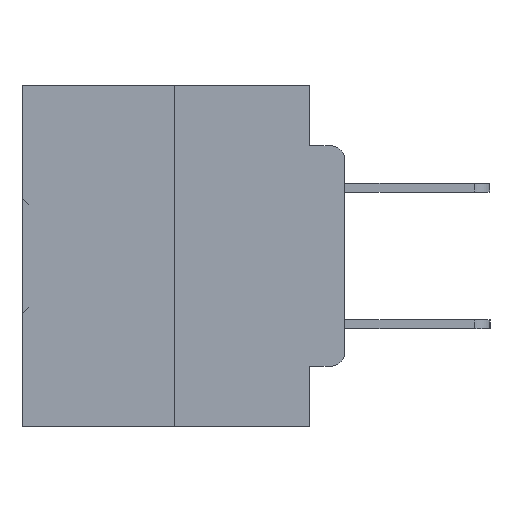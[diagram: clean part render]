
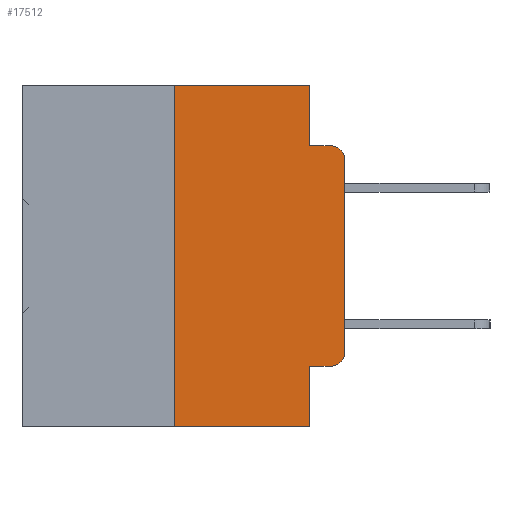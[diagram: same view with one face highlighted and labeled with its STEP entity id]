
A CAD part, left-side view. The second image highlights one B-rep face of the part: STEP entity #17512.
In plain terms, the highlighted planar face has unit normal (-1, 0, 0).
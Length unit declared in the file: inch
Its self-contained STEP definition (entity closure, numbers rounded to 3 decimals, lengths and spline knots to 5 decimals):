
#253 = VERTEX_POINT ( 'NONE', #17229 ) ;
#1044 = LINE ( 'NONE', #12478, #2604 ) ;
#1813 = DIRECTION ( 'NONE',  ( 0., 0., -1. ) ) ;
#1970 = VERTEX_POINT ( 'NONE', #19593 ) ;
#2037 = CARTESIAN_POINT ( 'NONE',  ( 0., 0.473, -0.5 ) ) ;
#2222 = DIRECTION ( 'NONE',  ( 0., 0., -1. ) ) ;
#2604 = VECTOR ( 'NONE', #35275, 39.37008 ) ;
#2745 = ORIENTED_EDGE ( 'NONE', *, *, #32824, .F. ) ;
#3114 = VECTOR ( 'NONE', #10471, 39.37008 ) ;
#3212 = CIRCLE ( 'NONE', #5008, 0.02 ) ;
#3658 = VERTEX_POINT ( 'NONE', #12360 ) ;
#3926 = CARTESIAN_POINT ( 'NONE',  ( 0., 0.473, 0. ) ) ;
#4075 = VERTEX_POINT ( 'NONE', #29695 ) ;
#4568 = VERTEX_POINT ( 'NONE', #26254 ) ;
#5008 = AXIS2_PLACEMENT_3D ( 'NONE', #9874, #18976, #12669 ) ;
#5252 = VECTOR ( 'NONE', #19465, 39.37008 ) ;
#5935 = CARTESIAN_POINT ( 'NONE',  ( 0., 0.051, 0. ) ) ;
#6738 = DIRECTION ( 'NONE',  ( 0., -1., 0. ) ) ;
#6985 = VERTEX_POINT ( 'NONE', #8319 ) ;
#7300 = ORIENTED_EDGE ( 'NONE', *, *, #29198, .F. ) ;
#7474 = DIRECTION ( 'NONE',  ( -1., 0., 0. ) ) ;
#7895 = DIRECTION ( 'NONE',  ( 0., -1., 0. ) ) ;
#8212 = LINE ( 'NONE', #5935, #25805 ) ;
#8319 = CARTESIAN_POINT ( 'NONE',  ( 0., 0., -0.1085 ) ) ;
#8607 = EDGE_CURVE ( 'NONE', #1970, #4568, #3212, .T. ) ;
#8662 = EDGE_CURVE ( 'NONE', #253, #34186, #1044, .T. ) ;
#9815 = AXIS2_PLACEMENT_3D ( 'NONE', #30672, #7474, #2222 ) ;
#9874 = CARTESIAN_POINT ( 'NONE',  ( 0., 0.02, -0.3915 ) ) ;
#10471 = DIRECTION ( 'NONE',  ( 0., -1., 0. ) ) ;
#11184 = VECTOR ( 'NONE', #6738, 39.37008 ) ;
#11772 = DIRECTION ( 'NONE',  ( 0., 0., 1. ) ) ;
#12360 = CARTESIAN_POINT ( 'NONE',  ( 0., 0.02, -0.0885 ) ) ;
#12478 = CARTESIAN_POINT ( 'NONE',  ( 0., 0.25, 0. ) ) ;
#12669 = DIRECTION ( 'NONE',  ( 0., 0., -1. ) ) ;
#12784 = CARTESIAN_POINT ( 'NONE',  ( 0., 0.051, -0.0885 ) ) ;
#13029 = VERTEX_POINT ( 'NONE', #31068 ) ;
#13443 = FACE_OUTER_BOUND ( 'NONE', #26329, .T. ) ;
#13804 = PLANE ( 'NONE',  #31922 ) ;
#14104 = ORIENTED_EDGE ( 'NONE', *, *, #8607, .T. ) ;
#14581 = ORIENTED_EDGE ( 'NONE', *, *, #24081, .F. ) ;
#15659 = CARTESIAN_POINT ( 'NONE',  ( 0., 0.051, 0. ) ) ;
#15830 = VERTEX_POINT ( 'NONE', #12784 ) ;
#16785 = EDGE_CURVE ( 'NONE', #13029, #1970, #22273, .T. ) ;
#17012 = LINE ( 'NONE', #17372, #36598 ) ;
#17229 = CARTESIAN_POINT ( 'NONE',  ( 0., 0.25, -0.5 ) ) ;
#17372 = CARTESIAN_POINT ( 'NONE',  ( 0., 0., 0. ) ) ;
#17512 = ADVANCED_FACE ( 'NONE', ( #13443 ), #13804, .F. ) ;
#18146 = CARTESIAN_POINT ( 'NONE',  ( 0., 0.25, 0. ) ) ;
#18416 = ORIENTED_EDGE ( 'NONE', *, *, #25282, .T. ) ;
#18439 = ORIENTED_EDGE ( 'NONE', *, *, #16785, .T. ) ;
#18799 = VERTEX_POINT ( 'NONE', #15659 ) ;
#18976 = DIRECTION ( 'NONE',  ( -1., 0., 0. ) ) ;
#19065 = VECTOR ( 'NONE', #27111, 39.37008 ) ;
#19465 = DIRECTION ( 'NONE',  ( 0., 0., -1. ) ) ;
#19593 = CARTESIAN_POINT ( 'NONE',  ( 0., 0.02, -0.4115 ) ) ;
#22273 = LINE ( 'NONE', #36890, #33662 ) ;
#22541 = CARTESIAN_POINT ( 'NONE',  ( 0., 0.473, 0. ) ) ;
#23745 = LINE ( 'NONE', #3926, #11184 ) ;
#24029 = EDGE_CURVE ( 'NONE', #253, #4075, #24663, .T. ) ;
#24081 = EDGE_CURVE ( 'NONE', #18799, #15830, #8212, .T. ) ;
#24663 = LINE ( 'NONE', #2037, #3114 ) ;
#25172 = DIRECTION ( 'NONE',  ( 1., 0., 0. ) ) ;
#25282 = EDGE_CURVE ( 'NONE', #6985, #3658, #28890, .T. ) ;
#25805 = VECTOR ( 'NONE', #28023, 39.37008 ) ;
#26254 = CARTESIAN_POINT ( 'NONE',  ( 0., 0., -0.3915 ) ) ;
#26329 = EDGE_LOOP ( 'NONE', ( #27714, #18416, #2745, #14581, #34530, #27811, #29169, #7300, #18439, #14104 ) ) ;
#27111 = DIRECTION ( 'NONE',  ( 0., -1., 0. ) ) ;
#27714 = ORIENTED_EDGE ( 'NONE', *, *, #36957, .T. ) ;
#27811 = ORIENTED_EDGE ( 'NONE', *, *, #8662, .F. ) ;
#28023 = DIRECTION ( 'NONE',  ( 0., 0., -1. ) ) ;
#28189 = EDGE_CURVE ( 'NONE', #34186, #18799, #23745, .T. ) ;
#28890 = CIRCLE ( 'NONE', #9815, 0.02 ) ;
#29169 = ORIENTED_EDGE ( 'NONE', *, *, #24029, .T. ) ;
#29198 = EDGE_CURVE ( 'NONE', #13029, #4075, #36526, .T. ) ;
#29695 = CARTESIAN_POINT ( 'NONE',  ( 0., 0.051, -0.5 ) ) ;
#29739 = LINE ( 'NONE', #29922, #19065 ) ;
#29922 = CARTESIAN_POINT ( 'NONE',  ( 0., 0.051, -0.0885 ) ) ;
#30672 = CARTESIAN_POINT ( 'NONE',  ( 0., 0.02, -0.1085 ) ) ;
#30904 = CARTESIAN_POINT ( 'NONE',  ( 0., 0.051, 0. ) ) ;
#31068 = CARTESIAN_POINT ( 'NONE',  ( 0., 0.051, -0.4115 ) ) ;
#31922 = AXIS2_PLACEMENT_3D ( 'NONE', #22541, #25172, #1813 ) ;
#32824 = EDGE_CURVE ( 'NONE', #15830, #3658, #29739, .T. ) ;
#33662 = VECTOR ( 'NONE', #7895, 39.37008 ) ;
#34186 = VERTEX_POINT ( 'NONE', #18146 ) ;
#34530 = ORIENTED_EDGE ( 'NONE', *, *, #28189, .F. ) ;
#35275 = DIRECTION ( 'NONE',  ( 0., 0., 1. ) ) ;
#36526 = LINE ( 'NONE', #30904, #5252 ) ;
#36598 = VECTOR ( 'NONE', #11772, 39.37008 ) ;
#36890 = CARTESIAN_POINT ( 'NONE',  ( 0., 0.051, -0.4115 ) ) ;
#36957 = EDGE_CURVE ( 'NONE', #4568, #6985, #17012, .T. ) ;
